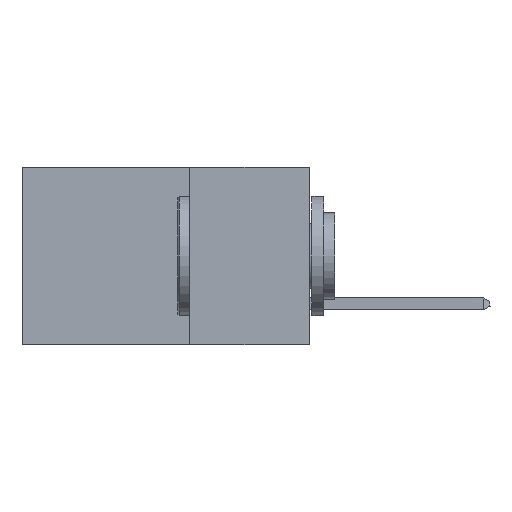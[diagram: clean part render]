
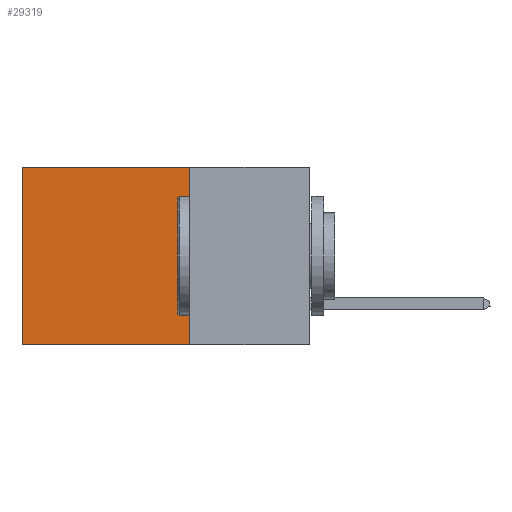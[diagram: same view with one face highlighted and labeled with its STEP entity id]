
A CAD part, left-side view. The second image highlights one B-rep face of the part: STEP entity #29319.
In plain terms, the highlighted planar face has unit normal (-1, 0, 0).
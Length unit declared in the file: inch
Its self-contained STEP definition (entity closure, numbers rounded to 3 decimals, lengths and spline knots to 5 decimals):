
#507 = VERTEX_POINT ( 'NONE', #24067 ) ;
#681 = CARTESIAN_POINT ( 'NONE',  ( 0.2875, 0.25, 0. ) ) ;
#4297 = CARTESIAN_POINT ( 'NONE',  ( 0.2875, 0.25, 0. ) ) ;
#4508 = EDGE_CURVE ( 'NONE', #4836, #14180, #6560, .T. ) ;
#4808 = CARTESIAN_POINT ( 'NONE',  ( 0.2875, 0.25, -0.37 ) ) ;
#4836 = VERTEX_POINT ( 'NONE', #4297 ) ;
#5489 = LINE ( 'NONE', #33916, #7641 ) ;
#5496 = EDGE_LOOP ( 'NONE', ( #10883, #25899, #9667, #19841 ) ) ;
#6560 = LINE ( 'NONE', #681, #23025 ) ;
#7641 = VECTOR ( 'NONE', #20058, 39.37008 ) ;
#9667 = ORIENTED_EDGE ( 'NONE', *, *, #31323, .F. ) ;
#10373 = VERTEX_POINT ( 'NONE', #31104 ) ;
#10883 = ORIENTED_EDGE ( 'NONE', *, *, #27439, .T. ) ;
#12064 = EDGE_CURVE ( 'NONE', #507, #10373, #15565, .T. ) ;
#12195 = CARTESIAN_POINT ( 'NONE',  ( 0.2875, 0.25, 0. ) ) ;
#12932 = VECTOR ( 'NONE', #16119, 39.37008 ) ;
#13333 = CARTESIAN_POINT ( 'NONE',  ( 0.2875, 0.6, 0. ) ) ;
#14180 = VERTEX_POINT ( 'NONE', #18467 ) ;
#15565 = LINE ( 'NONE', #4808, #12932 ) ;
#16119 = DIRECTION ( 'NONE',  ( 0., 1., 0. ) ) ;
#16170 = DIRECTION ( 'NONE',  ( 0., 0., -1. ) ) ;
#18467 = CARTESIAN_POINT ( 'NONE',  ( 0.2875, 0.6, 0. ) ) ;
#18508 = VECTOR ( 'NONE', #16170, 39.37008 ) ;
#19841 = ORIENTED_EDGE ( 'NONE', *, *, #4508, .T. ) ;
#20058 = DIRECTION ( 'NONE',  ( 0., 0., -1. ) ) ;
#20552 = FACE_OUTER_BOUND ( 'NONE', #5496, .T. ) ;
#20565 = DIRECTION ( 'NONE',  ( 0., 0., -1. ) ) ;
#23025 = VECTOR ( 'NONE', #23577, 39.37008 ) ;
#23577 = DIRECTION ( 'NONE',  ( 0., 1., 0. ) ) ;
#24067 = CARTESIAN_POINT ( 'NONE',  ( 0.2875, 0.25, -0.37 ) ) ;
#25899 = ORIENTED_EDGE ( 'NONE', *, *, #12064, .F. ) ;
#26310 = AXIS2_PLACEMENT_3D ( 'NONE', #12195, #31661, #20565 ) ;
#27439 = EDGE_CURVE ( 'NONE', #14180, #10373, #35907, .T. ) ;
#29319 = ADVANCED_FACE ( 'NONE', ( #20552 ), #34728, .F. ) ;
#31104 = CARTESIAN_POINT ( 'NONE',  ( 0.2875, 0.6, -0.37 ) ) ;
#31323 = EDGE_CURVE ( 'NONE', #4836, #507, #5489, .T. ) ;
#31661 = DIRECTION ( 'NONE',  ( 1., 0., 0. ) ) ;
#33916 = CARTESIAN_POINT ( 'NONE',  ( 0.2875, 0.25, 0. ) ) ;
#34728 = PLANE ( 'NONE',  #26310 ) ;
#35907 = LINE ( 'NONE', #13333, #18508 ) ;
